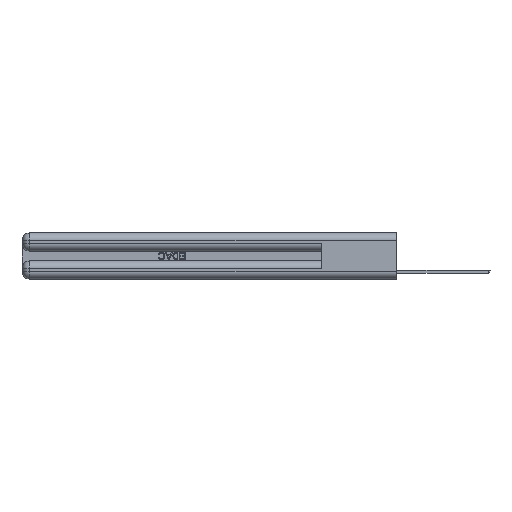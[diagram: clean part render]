
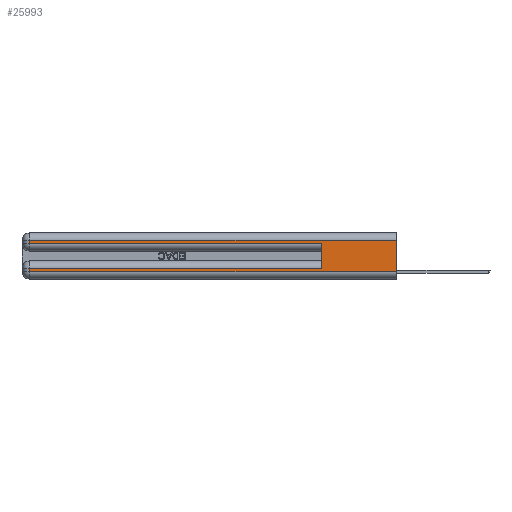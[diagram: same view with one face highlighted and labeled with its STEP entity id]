
A CAD part, left-side view. The second image highlights one B-rep face of the part: STEP entity #25993.
In plain terms, the highlighted planar face has unit normal (-1, 0, 0).
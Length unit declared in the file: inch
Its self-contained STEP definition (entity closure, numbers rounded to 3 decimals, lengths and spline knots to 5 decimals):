
#1672 = CARTESIAN_POINT ( 'NONE',  ( 0., 2.94, 0.085 ) ) ;
#2795 = VECTOR ( 'NONE', #24840, 39.37008 ) ;
#3578 = CARTESIAN_POINT ( 'NONE',  ( 0., 2.94, 0.06 ) ) ;
#4296 = VECTOR ( 'NONE', #19865, 39.37008 ) ;
#4905 = DIRECTION ( 'NONE',  ( 0., -1., 0. ) ) ;
#4931 = ORIENTED_EDGE ( 'NONE', *, *, #13466, .T. ) ;
#5091 = ORIENTED_EDGE ( 'NONE', *, *, #31038, .F. ) ;
#5268 = ORIENTED_EDGE ( 'NONE', *, *, #7208, .T. ) ;
#5730 = DIRECTION ( 'NONE',  ( 0., -1., 0. ) ) ;
#6298 = CARTESIAN_POINT ( 'NONE',  ( 0., 2.94, 0.37 ) ) ;
#7208 = EDGE_CURVE ( 'NONE', #11358, #31472, #21330, .T. ) ;
#7952 = ORIENTED_EDGE ( 'NONE', *, *, #14663, .T. ) ;
#8062 = AXIS2_PLACEMENT_3D ( 'NONE', #10682, #28497, #23126 ) ;
#8247 = LINE ( 'NONE', #28736, #25382 ) ;
#9185 = CARTESIAN_POINT ( 'NONE',  ( 0., 0., 0.06 ) ) ;
#9214 = LINE ( 'NONE', #32220, #2795 ) ;
#9734 = CARTESIAN_POINT ( 'NONE',  ( 0., 0.6, 0.145 ) ) ;
#10045 = CARTESIAN_POINT ( 'NONE',  ( 0., 2.94, 0.285 ) ) ;
#10090 = LINE ( 'NONE', #15142, #4296 ) ;
#10215 = VECTOR ( 'NONE', #25751, 39.37008 ) ;
#10330 = EDGE_CURVE ( 'NONE', #25641, #25042, #21423, .T. ) ;
#10682 = CARTESIAN_POINT ( 'NONE',  ( 0., 0., 0.37 ) ) ;
#11018 = ORIENTED_EDGE ( 'NONE', *, *, #30617, .T. ) ;
#11166 = DIRECTION ( 'NONE',  ( 0., 0., -1. ) ) ;
#11358 = VERTEX_POINT ( 'NONE', #26634 ) ;
#11591 = VERTEX_POINT ( 'NONE', #3578 ) ;
#12869 = FACE_OUTER_BOUND ( 'NONE', #27009, .T. ) ;
#12965 = CARTESIAN_POINT ( 'NONE',  ( 0., 0., 0.31 ) ) ;
#13466 = EDGE_CURVE ( 'NONE', #25042, #22764, #8247, .T. ) ;
#14415 = ORIENTED_EDGE ( 'NONE', *, *, #31491, .F. ) ;
#14663 = EDGE_CURVE ( 'NONE', #16941, #25641, #9214, .T. ) ;
#15142 = CARTESIAN_POINT ( 'NONE',  ( 0., 2.94, 0.37 ) ) ;
#15579 = VECTOR ( 'NONE', #22336, 39.37008 ) ;
#16353 = VERTEX_POINT ( 'NONE', #9185 ) ;
#16570 = ORIENTED_EDGE ( 'NONE', *, *, #10330, .T. ) ;
#16941 = VERTEX_POINT ( 'NONE', #12965 ) ;
#17676 = LINE ( 'NONE', #27917, #18787 ) ;
#18787 = VECTOR ( 'NONE', #4905, 39.37008 ) ;
#19865 = DIRECTION ( 'NONE',  ( 0., 0., -1. ) ) ;
#20471 = VECTOR ( 'NONE', #11166, 39.37008 ) ;
#20771 = PLANE ( 'NONE',  #8062 ) ;
#21330 = LINE ( 'NONE', #31396, #32691 ) ;
#21423 = LINE ( 'NONE', #6298, #20471 ) ;
#22088 = CARTESIAN_POINT ( 'NONE',  ( 0., 2.94, 0.31 ) ) ;
#22136 = CARTESIAN_POINT ( 'NONE',  ( 0., 0., 0.37 ) ) ;
#22336 = DIRECTION ( 'NONE',  ( 0., 0., 1. ) ) ;
#22764 = VERTEX_POINT ( 'NONE', #24265 ) ;
#23126 = DIRECTION ( 'NONE',  ( 0., 0., -1. ) ) ;
#23240 = LINE ( 'NONE', #22136, #10215 ) ;
#24265 = CARTESIAN_POINT ( 'NONE',  ( 0., 0.6, 0.285 ) ) ;
#24840 = DIRECTION ( 'NONE',  ( 0., 1., 0. ) ) ;
#25042 = VERTEX_POINT ( 'NONE', #10045 ) ;
#25382 = VECTOR ( 'NONE', #5730, 39.37008 ) ;
#25641 = VERTEX_POINT ( 'NONE', #22088 ) ;
#25751 = DIRECTION ( 'NONE',  ( 0., 0., -1. ) ) ;
#25993 = ADVANCED_FACE ( 'NONE', ( #12869 ), #20771, .F. ) ;
#26634 = CARTESIAN_POINT ( 'NONE',  ( 0., 0.6, 0.085 ) ) ;
#27009 = EDGE_LOOP ( 'NONE', ( #14415, #7952, #16570, #4931, #5091, #5268, #30318, #11018 ) ) ;
#27917 = CARTESIAN_POINT ( 'NONE',  ( 0., 0., 0.06 ) ) ;
#28386 = DIRECTION ( 'NONE',  ( 0., 1., 0. ) ) ;
#28497 = DIRECTION ( 'NONE',  ( 1., 0., 0. ) ) ;
#28736 = CARTESIAN_POINT ( 'NONE',  ( 0., 0., 0.285 ) ) ;
#30052 = LINE ( 'NONE', #9734, #15579 ) ;
#30318 = ORIENTED_EDGE ( 'NONE', *, *, #30622, .T. ) ;
#30617 = EDGE_CURVE ( 'NONE', #11591, #16353, #17676, .T. ) ;
#30622 = EDGE_CURVE ( 'NONE', #31472, #11591, #10090, .T. ) ;
#31038 = EDGE_CURVE ( 'NONE', #11358, #22764, #30052, .T. ) ;
#31396 = CARTESIAN_POINT ( 'NONE',  ( 0., 0., 0.085 ) ) ;
#31472 = VERTEX_POINT ( 'NONE', #1672 ) ;
#31491 = EDGE_CURVE ( 'NONE', #16941, #16353, #23240, .T. ) ;
#32220 = CARTESIAN_POINT ( 'NONE',  ( 0., 0., 0.31 ) ) ;
#32691 = VECTOR ( 'NONE', #28386, 39.37008 ) ;
